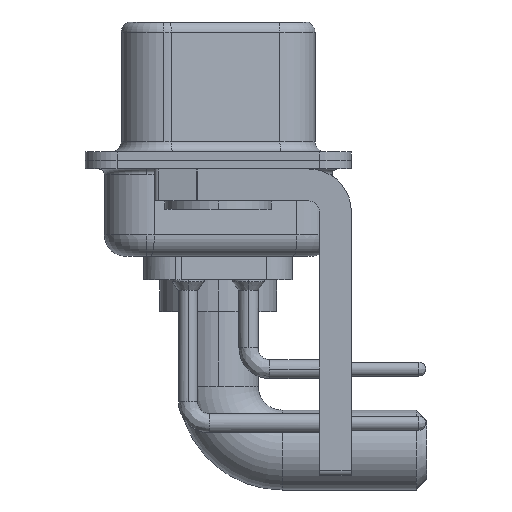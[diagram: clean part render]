
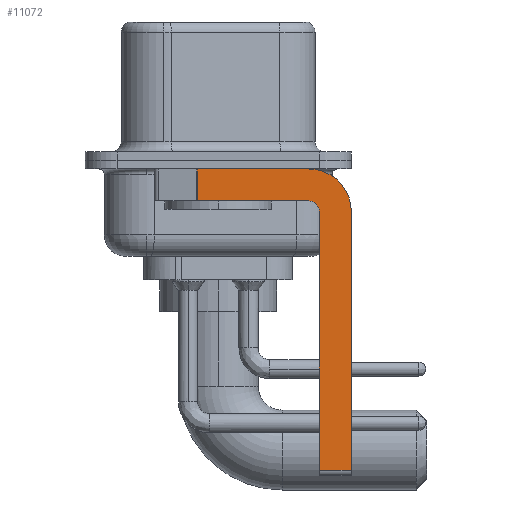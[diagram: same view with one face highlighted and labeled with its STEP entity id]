
A CAD part, left-side view. The second image highlights one B-rep face of the part: STEP entity #11072.
In plain terms, the highlighted planar face has unit normal (-1, 0, 0).
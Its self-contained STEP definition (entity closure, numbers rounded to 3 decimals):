
#167 = DIRECTION ( 'NONE',  ( 0., 0., -1. ) ) ;
#813 = ORIENTED_EDGE ( 'NONE', *, *, #23036, .F. ) ;
#937 = VECTOR ( 'NONE', #17945, 1000. ) ;
#986 = DIRECTION ( 'NONE',  ( 0., -1., 0. ) ) ;
#1142 = CARTESIAN_POINT ( 'NONE',  ( -2.9, -4.75, -2.4 ) ) ;
#1492 = CARTESIAN_POINT ( 'NONE',  ( -2.9, 0.978, -1.9 ) ) ;
#1507 = VERTEX_POINT ( 'NONE', #2766 ) ;
#1561 = EDGE_CURVE ( 'NONE', #17542, #21042, #13227, .T. ) ;
#2766 = CARTESIAN_POINT ( 'NONE',  ( -2.9, -6.25, -2.4 ) ) ;
#3440 = DIRECTION ( 'NONE',  ( 1., 0., 0. ) ) ;
#5040 = EDGE_LOOP ( 'NONE', ( #7751, #10390, #813, #18827, #13367, #21955, #14844, #15500 ) ) ;
#5107 = CARTESIAN_POINT ( 'NONE',  ( -2.9, -4.25, -2.4 ) ) ;
#5191 = FACE_OUTER_BOUND ( 'NONE', #5040, .T. ) ;
#5362 = VECTOR ( 'NONE', #10653, 1000. ) ;
#5945 = CARTESIAN_POINT ( 'NONE',  ( -2.9, 0.978, -0.4 ) ) ;
#6006 = CIRCLE ( 'NONE', #7492, 2. ) ;
#6740 = DIRECTION ( 'NONE',  ( 1., 0., 0. ) ) ;
#7195 = VERTEX_POINT ( 'NONE', #14994 ) ;
#7492 = AXIS2_PLACEMENT_3D ( 'NONE', #5107, #6740, #19496 ) ;
#7516 = CARTESIAN_POINT ( 'NONE',  ( -2.9, -4.25, -1.9 ) ) ;
#7615 = LINE ( 'NONE', #17835, #937 ) ;
#7751 = ORIENTED_EDGE ( 'NONE', *, *, #21143, .F. ) ;
#9189 = DIRECTION ( 'NONE',  ( 0., 0., -1. ) ) ;
#9675 = EDGE_CURVE ( 'NONE', #12873, #17542, #7615, .T. ) ;
#9816 = EDGE_CURVE ( 'NONE', #1507, #15151, #14309, .T. ) ;
#9859 = CARTESIAN_POINT ( 'NONE',  ( -2.9, 3., -0.4 ) ) ;
#10005 = EDGE_CURVE ( 'NONE', #12873, #15151, #17219, .T. ) ;
#10341 = CARTESIAN_POINT ( 'NONE',  ( -2.9, -4.25, -2.4 ) ) ;
#10390 = ORIENTED_EDGE ( 'NONE', *, *, #14461, .T. ) ;
#10653 = DIRECTION ( 'NONE',  ( 0., 1., 0. ) ) ;
#10884 = LINE ( 'NONE', #19780, #5362 ) ;
#11072 = ADVANCED_FACE ( 'NONE', ( #5191 ), #13738, .F. ) ;
#12873 = VERTEX_POINT ( 'NONE', #21359 ) ;
#12919 = VECTOR ( 'NONE', #13821, 1000. ) ;
#13129 = VERTEX_POINT ( 'NONE', #18762 ) ;
#13227 = CIRCLE ( 'NONE', #16238, 0.5 ) ;
#13367 = ORIENTED_EDGE ( 'NONE', *, *, #9675, .F. ) ;
#13738 = PLANE ( 'NONE',  #20809 ) ;
#13821 = DIRECTION ( 'NONE',  ( 0., -1., 0. ) ) ;
#13857 = VECTOR ( 'NONE', #9189, 1000. ) ;
#14309 = LINE ( 'NONE', #16529, #19264 ) ;
#14402 = EDGE_CURVE ( 'NONE', #7195, #1507, #6006, .T. ) ;
#14461 = EDGE_CURVE ( 'NONE', #16293, #13129, #17513, .T. ) ;
#14844 = ORIENTED_EDGE ( 'NONE', *, *, #9816, .F. ) ;
#14936 = CARTESIAN_POINT ( 'NONE',  ( -2.9, -4.25, -2.4 ) ) ;
#14994 = CARTESIAN_POINT ( 'NONE',  ( -2.9, -4.25, -0.4 ) ) ;
#15151 = VERTEX_POINT ( 'NONE', #20278 ) ;
#15177 = DIRECTION ( 'NONE',  ( -1., 0., 0. ) ) ;
#15500 = ORIENTED_EDGE ( 'NONE', *, *, #14402, .F. ) ;
#15622 = DIRECTION ( 'NONE',  ( 0., 0., -1. ) ) ;
#15789 = VECTOR ( 'NONE', #986, 1000. ) ;
#16238 = AXIS2_PLACEMENT_3D ( 'NONE', #14936, #15177, #22318 ) ;
#16293 = VERTEX_POINT ( 'NONE', #5945 ) ;
#16529 = CARTESIAN_POINT ( 'NONE',  ( -2.9, -6.25, -2.4 ) ) ;
#17219 = LINE ( 'NONE', #20730, #12919 ) ;
#17513 = LINE ( 'NONE', #1492, #13857 ) ;
#17542 = VERTEX_POINT ( 'NONE', #1142 ) ;
#17835 = CARTESIAN_POINT ( 'NONE',  ( -2.9, -4.75, -14.8 ) ) ;
#17945 = DIRECTION ( 'NONE',  ( 0., 0., 1. ) ) ;
#18762 = CARTESIAN_POINT ( 'NONE',  ( -2.9, 0.978, -1.9 ) ) ;
#18827 = ORIENTED_EDGE ( 'NONE', *, *, #1561, .F. ) ;
#18883 = LINE ( 'NONE', #9859, #15789 ) ;
#19264 = VECTOR ( 'NONE', #167, 1000. ) ;
#19496 = DIRECTION ( 'NONE',  ( 0., 0., -1. ) ) ;
#19780 = CARTESIAN_POINT ( 'NONE',  ( -2.9, -4.25, -1.9 ) ) ;
#20278 = CARTESIAN_POINT ( 'NONE',  ( -2.9, -6.25, -14.55 ) ) ;
#20730 = CARTESIAN_POINT ( 'NONE',  ( -2.9, -4.25, -14.55 ) ) ;
#20809 = AXIS2_PLACEMENT_3D ( 'NONE', #10341, #3440, #15622 ) ;
#21042 = VERTEX_POINT ( 'NONE', #7516 ) ;
#21143 = EDGE_CURVE ( 'NONE', #16293, #7195, #18883, .T. ) ;
#21359 = CARTESIAN_POINT ( 'NONE',  ( -2.9, -4.75, -14.55 ) ) ;
#21955 = ORIENTED_EDGE ( 'NONE', *, *, #10005, .T. ) ;
#22318 = DIRECTION ( 'NONE',  ( 0., 0., 1. ) ) ;
#23036 = EDGE_CURVE ( 'NONE', #21042, #13129, #10884, .T. ) ;
